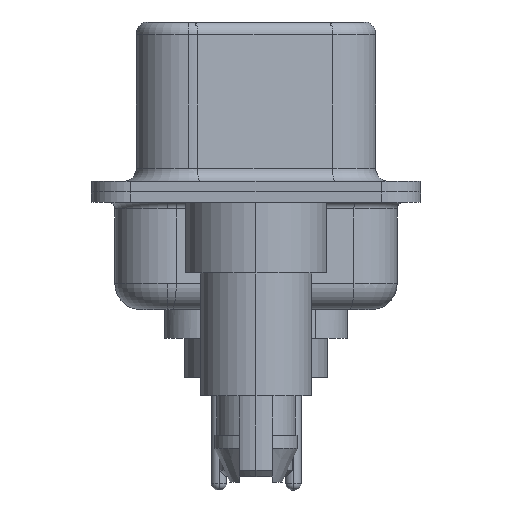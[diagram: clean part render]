
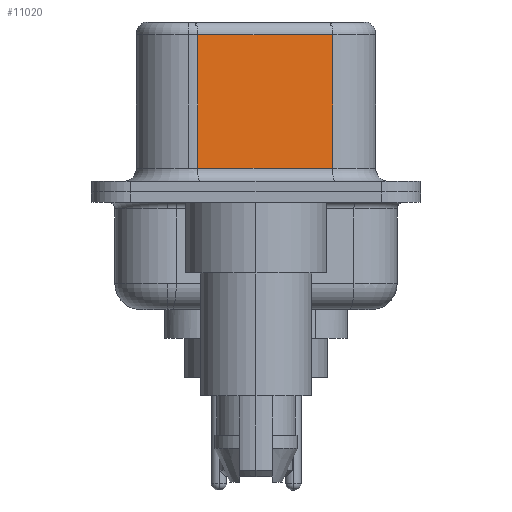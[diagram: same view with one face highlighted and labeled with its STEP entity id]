
A CAD part, left-side view. The second image highlights one B-rep face of the part: STEP entity #11020.
In plain terms, the highlighted planar face has unit normal (-0.985, -0.174, 0).
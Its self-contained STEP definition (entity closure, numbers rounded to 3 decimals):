
#693 = AXIS2_PLACEMENT_3D ( 'NONE', #17831, #7464, #19574 ) ;
#1326 = VECTOR ( 'NONE', #3632, 1000. ) ;
#1720 = EDGE_CURVE ( 'NONE', #21454, #17955, #19653, .T. ) ;
#3062 = ORIENTED_EDGE ( 'NONE', *, *, #7915, .T. ) ;
#3445 = CARTESIAN_POINT ( 'NONE',  ( 3.67, 2.233, 0.9 ) ) ;
#3632 = DIRECTION ( 'NONE',  ( 0., 0., -1. ) ) ;
#4233 = CARTESIAN_POINT ( 'NONE',  ( 4.58, -2.927, 6.52 ) ) ;
#5131 = FACE_OUTER_BOUND ( 'NONE', #16363, .T. ) ;
#6007 = DIRECTION ( 'NONE',  ( 0., 0., -1. ) ) ;
#6239 = ORIENTED_EDGE ( 'NONE', *, *, #1720, .T. ) ;
#6457 = LINE ( 'NONE', #4233, #10566 ) ;
#7464 = DIRECTION ( 'NONE',  ( 0.985, 0.174, 0. ) ) ;
#7915 = EDGE_CURVE ( 'NONE', #16260, #21454, #8249, .T. ) ;
#7981 = EDGE_CURVE ( 'NONE', #17955, #8417, #12784, .T. ) ;
#8249 = LINE ( 'NONE', #14216, #21485 ) ;
#8417 = VERTEX_POINT ( 'NONE', #19219 ) ;
#9903 = EDGE_CURVE ( 'NONE', #16260, #8417, #6457, .T. ) ;
#10566 = VECTOR ( 'NONE', #6007, 1000. ) ;
#11020 = ADVANCED_FACE ( 'NONE', ( #5131 ), #16064, .F. ) ;
#11455 = ORIENTED_EDGE ( 'NONE', *, *, #9903, .F. ) ;
#11836 = DIRECTION ( 'NONE',  ( 0.174, -0.985, 0. ) ) ;
#12114 = CARTESIAN_POINT ( 'NONE',  ( 4.58, -2.927, 0.9 ) ) ;
#12784 = LINE ( 'NONE', #12114, #16308 ) ;
#13282 = CARTESIAN_POINT ( 'NONE',  ( 3.67, 2.233, 6.52 ) ) ;
#14216 = CARTESIAN_POINT ( 'NONE',  ( 4.58, -2.927, 6.02 ) ) ;
#15034 = ORIENTED_EDGE ( 'NONE', *, *, #7981, .T. ) ;
#15784 = CARTESIAN_POINT ( 'NONE',  ( 4.58, -2.927, 6.02 ) ) ;
#16064 = PLANE ( 'NONE',  #693 ) ;
#16260 = VERTEX_POINT ( 'NONE', #15784 ) ;
#16308 = VECTOR ( 'NONE', #11836, 1000. ) ;
#16363 = EDGE_LOOP ( 'NONE', ( #11455, #3062, #6239, #15034 ) ) ;
#17831 = CARTESIAN_POINT ( 'NONE',  ( 4.58, -2.927, 6.52 ) ) ;
#17955 = VERTEX_POINT ( 'NONE', #3445 ) ;
#19026 = DIRECTION ( 'NONE',  ( -0.174, 0.985, 0. ) ) ;
#19219 = CARTESIAN_POINT ( 'NONE',  ( 4.58, -2.927, 0.9 ) ) ;
#19574 = DIRECTION ( 'NONE',  ( -0.174, 0.985, 0. ) ) ;
#19653 = LINE ( 'NONE', #13282, #1326 ) ;
#20934 = CARTESIAN_POINT ( 'NONE',  ( 3.67, 2.233, 6.02 ) ) ;
#21454 = VERTEX_POINT ( 'NONE', #20934 ) ;
#21485 = VECTOR ( 'NONE', #19026, 1000. ) ;
